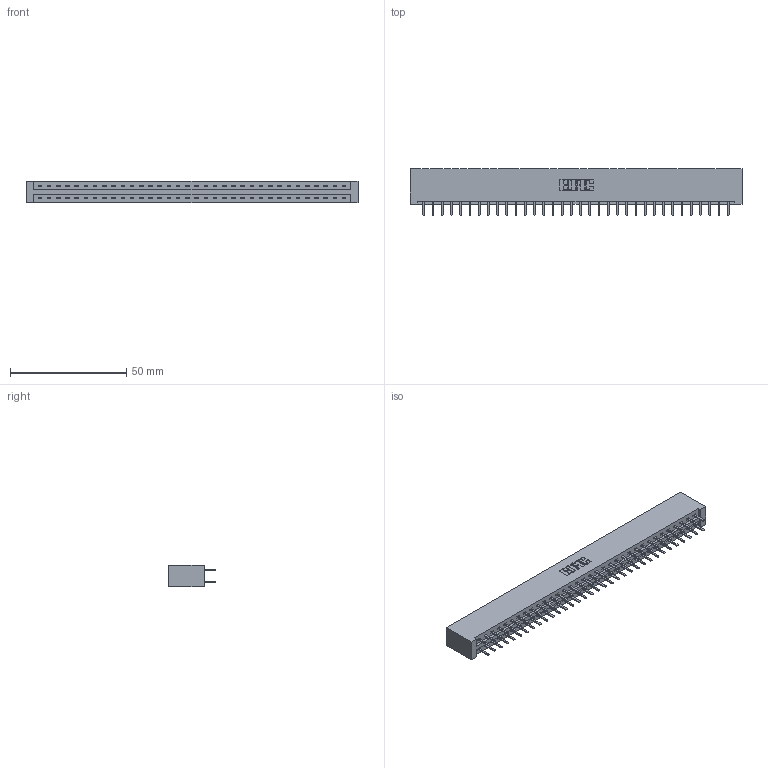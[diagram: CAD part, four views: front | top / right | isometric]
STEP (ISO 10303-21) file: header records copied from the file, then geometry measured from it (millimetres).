
FILE_DESCRIPTION (( 'STEP AP203' ), '1' );
FILE_NAME ('337-068-520-201.STEP', '2019-10-09T23:52:39', ( '' ), ( '' ), 'SwSTEP 2.0', 'SolidWorks 2016', '' );
FILE_SCHEMA (( 'CONFIG_CONTROL_DESIGN' ));
Length unit declared in the file: inch
Products named in the file (3): 345-292-001_345-293-120; 337-068-520-201; 337 Part_No Mounting Lugs
Assembly tree (69 placements, depth 2):
  337-068-520-201
    337 Part_No Mounting Lugs
    345-292-001_345-293-120  x68
Bounding box: 142.6 x 20.02 x 9.4 mm (x, y, z)
Volume: 15652.2 mm3; surface area: 17588 mm2
Topology: 69 solids, 69 shells, 4050 faces, 11779 edges, 7670 vertices
Faces by surface type: plane 2786, cylinder 1264
Entity records: 27233 total; most frequent: CARTESIAN_POINT 4606, ORIENTED_EDGE 4530, DIRECTION 3913, EDGE_CURVE 2265, LINE 2141, VECTOR 2141, VERTEX_POINT 1506, AXIS2_PLACEMENT_3D 886
